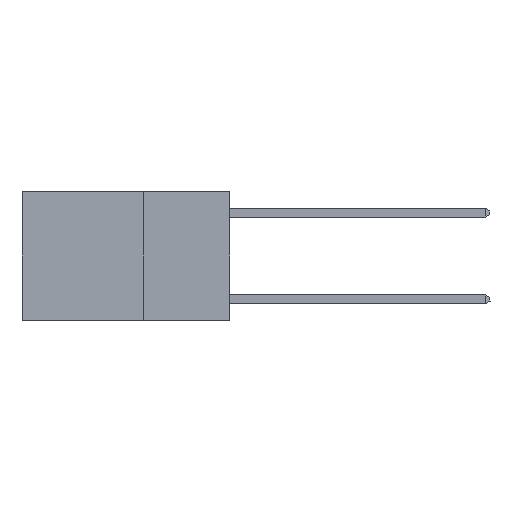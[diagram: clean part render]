
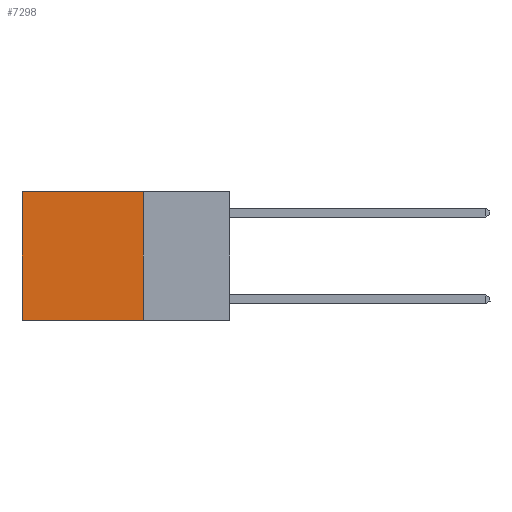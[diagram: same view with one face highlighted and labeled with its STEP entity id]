
A CAD part, left-side view. The second image highlights one B-rep face of the part: STEP entity #7298.
In plain terms, the highlighted planar face has unit normal (-1, 0, 0).
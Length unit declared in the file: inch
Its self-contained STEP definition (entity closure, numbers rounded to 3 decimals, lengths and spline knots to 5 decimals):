
#539 = ORIENTED_EDGE ( 'NONE', *, *, #719, .T. ) ;
#719 = EDGE_CURVE ( 'NONE', #14261, #13357, #17026, .T. ) ;
#1233 = EDGE_CURVE ( 'NONE', #6542, #13357, #16495, .T. ) ;
#1519 = CARTESIAN_POINT ( 'NONE',  ( 0.2625, 0.25, 0. ) ) ;
#1948 = CARTESIAN_POINT ( 'NONE',  ( 0.2625, 0.25, -0.37 ) ) ;
#2699 = LINE ( 'NONE', #1519, #14783 ) ;
#3121 = CARTESIAN_POINT ( 'NONE',  ( 0.2625, 0.25, 0. ) ) ;
#3382 = VECTOR ( 'NONE', #7757, 39.37008 ) ;
#4250 = EDGE_LOOP ( 'NONE', ( #539, #5448, #17817, #16074 ) ) ;
#4278 = AXIS2_PLACEMENT_3D ( 'NONE', #4990, #6655, #18086 ) ;
#4424 = CARTESIAN_POINT ( 'NONE',  ( 0.2625, 0.25, -0.37 ) ) ;
#4451 = EDGE_CURVE ( 'NONE', #4687, #14261, #18565, .T. ) ;
#4687 = VERTEX_POINT ( 'NONE', #18242 ) ;
#4990 = CARTESIAN_POINT ( 'NONE',  ( 0.2625, 0.25, 0. ) ) ;
#5448 = ORIENTED_EDGE ( 'NONE', *, *, #1233, .F. ) ;
#6130 = DIRECTION ( 'NONE',  ( 0., 0., -1. ) ) ;
#6542 = VERTEX_POINT ( 'NONE', #4424 ) ;
#6655 = DIRECTION ( 'NONE',  ( 1., 0., 0. ) ) ;
#7298 = ADVANCED_FACE ( 'NONE', ( #14614 ), #14797, .F. ) ;
#7757 = DIRECTION ( 'NONE',  ( 0., 1., 0. ) ) ;
#10726 = CARTESIAN_POINT ( 'NONE',  ( 0.2625, 0.6, -0.37 ) ) ;
#12709 = VECTOR ( 'NONE', #6130, 39.37008 ) ;
#13013 = DIRECTION ( 'NONE',  ( 0., 1., 0. ) ) ;
#13031 = EDGE_CURVE ( 'NONE', #4687, #6542, #2699, .T. ) ;
#13181 = DIRECTION ( 'NONE',  ( 0., 0., -1. ) ) ;
#13357 = VERTEX_POINT ( 'NONE', #10726 ) ;
#14261 = VERTEX_POINT ( 'NONE', #16176 ) ;
#14614 = FACE_OUTER_BOUND ( 'NONE', #4250, .T. ) ;
#14783 = VECTOR ( 'NONE', #13181, 39.37008 ) ;
#14797 = PLANE ( 'NONE',  #4278 ) ;
#16074 = ORIENTED_EDGE ( 'NONE', *, *, #4451, .T. ) ;
#16176 = CARTESIAN_POINT ( 'NONE',  ( 0.2625, 0.6, 0. ) ) ;
#16495 = LINE ( 'NONE', #1948, #3382 ) ;
#16794 = CARTESIAN_POINT ( 'NONE',  ( 0.2625, 0.6, 0. ) ) ;
#17026 = LINE ( 'NONE', #16794, #12709 ) ;
#17817 = ORIENTED_EDGE ( 'NONE', *, *, #13031, .F. ) ;
#18050 = VECTOR ( 'NONE', #13013, 39.37008 ) ;
#18086 = DIRECTION ( 'NONE',  ( 0., 0., -1. ) ) ;
#18242 = CARTESIAN_POINT ( 'NONE',  ( 0.2625, 0.25, 0. ) ) ;
#18565 = LINE ( 'NONE', #3121, #18050 ) ;
